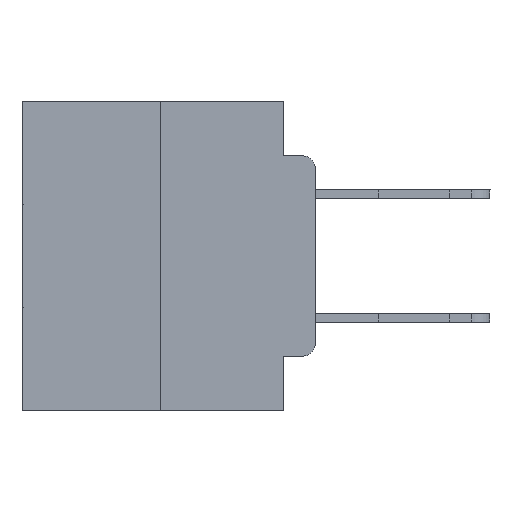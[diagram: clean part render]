
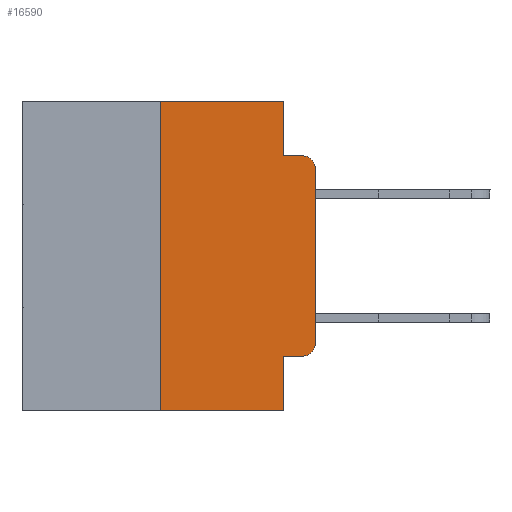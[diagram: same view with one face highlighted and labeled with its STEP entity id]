
A CAD part, left-side view. The second image highlights one B-rep face of the part: STEP entity #16590.
In plain terms, the highlighted planar face has unit normal (-1, 0, 0).
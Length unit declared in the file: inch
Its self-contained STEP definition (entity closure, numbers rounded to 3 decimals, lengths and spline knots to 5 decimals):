
#237 = DIRECTION ( 'NONE',  ( 0., 0., 1. ) ) ;
#585 = CARTESIAN_POINT ( 'NONE',  ( 0., 0.473, 0. ) ) ;
#592 = ORIENTED_EDGE ( 'NONE', *, *, #7788, .T. ) ;
#668 = VERTEX_POINT ( 'NONE', #2514 ) ;
#1977 = VERTEX_POINT ( 'NONE', #4377 ) ;
#2514 = CARTESIAN_POINT ( 'NONE',  ( 0., 0.051, 0. ) ) ;
#2603 = DIRECTION ( 'NONE',  ( 0., -1., 0. ) ) ;
#3077 = ORIENTED_EDGE ( 'NONE', *, *, #17697, .F. ) ;
#4150 = VECTOR ( 'NONE', #15888, 39.37008 ) ;
#4196 = ORIENTED_EDGE ( 'NONE', *, *, #24489, .F. ) ;
#4325 = CARTESIAN_POINT ( 'NONE',  ( 0., 0.051, -0.4115 ) ) ;
#4377 = CARTESIAN_POINT ( 'NONE',  ( 0., 0.25, -0.5 ) ) ;
#4650 = CARTESIAN_POINT ( 'NONE',  ( 0., 0., -0.1085 ) ) ;
#4877 = VERTEX_POINT ( 'NONE', #4325 ) ;
#4922 = LINE ( 'NONE', #20144, #4150 ) ;
#5727 = VERTEX_POINT ( 'NONE', #19335 ) ;
#6522 = DIRECTION ( 'NONE',  ( 0., 0., 1. ) ) ;
#6917 = LINE ( 'NONE', #19869, #20820 ) ;
#7224 = CARTESIAN_POINT ( 'NONE',  ( 0., 0.051, 0. ) ) ;
#7379 = DIRECTION ( 'NONE',  ( 0., 0., -1. ) ) ;
#7439 = CARTESIAN_POINT ( 'NONE',  ( 0., 0.02, -0.4115 ) ) ;
#7537 = EDGE_CURVE ( 'NONE', #4877, #9362, #4922, .T. ) ;
#7606 = CARTESIAN_POINT ( 'NONE',  ( 0., 0.473, -0.5 ) ) ;
#7788 = EDGE_CURVE ( 'NONE', #1977, #18421, #7886, .T. ) ;
#7886 = LINE ( 'NONE', #7606, #14644 ) ;
#8038 = DIRECTION ( 'NONE',  ( 1., 0., 0. ) ) ;
#8735 = EDGE_LOOP ( 'NONE', ( #16158, #27619, #15827, #17125, #17942, #3077, #592, #4196, #11547, #19178 ) ) ;
#9145 = CARTESIAN_POINT ( 'NONE',  ( 0., 0.051, -0.0885 ) ) ;
#9362 = VERTEX_POINT ( 'NONE', #7439 ) ;
#10074 = AXIS2_PLACEMENT_3D ( 'NONE', #19563, #8038, #23288 ) ;
#10873 = FACE_OUTER_BOUND ( 'NONE', #8735, .T. ) ;
#11146 = AXIS2_PLACEMENT_3D ( 'NONE', #19406, #27556, #17004 ) ;
#11332 = EDGE_CURVE ( 'NONE', #9362, #27834, #20157, .T. ) ;
#11547 = ORIENTED_EDGE ( 'NONE', *, *, #7537, .T. ) ;
#11781 = LINE ( 'NONE', #7224, #18985 ) ;
#12015 = VECTOR ( 'NONE', #14668, 39.37008 ) ;
#12826 = LINE ( 'NONE', #19213, #12015 ) ;
#12827 = CARTESIAN_POINT ( 'NONE',  ( 0., 0.02, -0.3915 ) ) ;
#12895 = PLANE ( 'NONE',  #10074 ) ;
#13830 = LINE ( 'NONE', #585, #20642 ) ;
#14644 = VECTOR ( 'NONE', #24995, 39.37008 ) ;
#14668 = DIRECTION ( 'NONE',  ( 0., 0., -1. ) ) ;
#15209 = VERTEX_POINT ( 'NONE', #23945 ) ;
#15827 = ORIENTED_EDGE ( 'NONE', *, *, #17400, .F. ) ;
#15888 = DIRECTION ( 'NONE',  ( 0., -1., 0. ) ) ;
#16083 = AXIS2_PLACEMENT_3D ( 'NONE', #12827, #21492, #28055 ) ;
#16158 = ORIENTED_EDGE ( 'NONE', *, *, #24740, .T. ) ;
#16590 = ADVANCED_FACE ( 'NONE', ( #10873 ), #12895, .F. ) ;
#16642 = VERTEX_POINT ( 'NONE', #24550 ) ;
#17004 = DIRECTION ( 'NONE',  ( 0., 0., -1. ) ) ;
#17076 = CARTESIAN_POINT ( 'NONE',  ( 0., 0.25, 0. ) ) ;
#17125 = ORIENTED_EDGE ( 'NONE', *, *, #19511, .F. ) ;
#17400 = EDGE_CURVE ( 'NONE', #16642, #5727, #26253, .T. ) ;
#17697 = EDGE_CURVE ( 'NONE', #1977, #15209, #19478, .T. ) ;
#17942 = ORIENTED_EDGE ( 'NONE', *, *, #20484, .F. ) ;
#18421 = VERTEX_POINT ( 'NONE', #26441 ) ;
#18985 = VECTOR ( 'NONE', #7379, 39.37008 ) ;
#19178 = ORIENTED_EDGE ( 'NONE', *, *, #11332, .T. ) ;
#19213 = CARTESIAN_POINT ( 'NONE',  ( 0., 0.051, 0. ) ) ;
#19335 = CARTESIAN_POINT ( 'NONE',  ( 0., 0.02, -0.0885 ) ) ;
#19406 = CARTESIAN_POINT ( 'NONE',  ( 0., 0.02, -0.1085 ) ) ;
#19478 = LINE ( 'NONE', #17076, #25613 ) ;
#19511 = EDGE_CURVE ( 'NONE', #668, #16642, #12826, .T. ) ;
#19563 = CARTESIAN_POINT ( 'NONE',  ( 0., 0.473, 0. ) ) ;
#19869 = CARTESIAN_POINT ( 'NONE',  ( 0., 0., 0. ) ) ;
#20089 = DIRECTION ( 'NONE',  ( 0., -1., 0. ) ) ;
#20144 = CARTESIAN_POINT ( 'NONE',  ( 0., 0.051, -0.4115 ) ) ;
#20157 = CIRCLE ( 'NONE', #16083, 0.02 ) ;
#20484 = EDGE_CURVE ( 'NONE', #15209, #668, #13830, .T. ) ;
#20642 = VECTOR ( 'NONE', #20089, 39.37008 ) ;
#20820 = VECTOR ( 'NONE', #237, 39.37008 ) ;
#21292 = VERTEX_POINT ( 'NONE', #4650 ) ;
#21492 = DIRECTION ( 'NONE',  ( -1., 0., 0. ) ) ;
#22249 = EDGE_CURVE ( 'NONE', #21292, #5727, #24811, .T. ) ;
#23288 = DIRECTION ( 'NONE',  ( 0., 0., -1. ) ) ;
#23945 = CARTESIAN_POINT ( 'NONE',  ( 0., 0.25, 0. ) ) ;
#24489 = EDGE_CURVE ( 'NONE', #4877, #18421, #11781, .T. ) ;
#24550 = CARTESIAN_POINT ( 'NONE',  ( 0., 0.051, -0.0885 ) ) ;
#24691 = VECTOR ( 'NONE', #2603, 39.37008 ) ;
#24740 = EDGE_CURVE ( 'NONE', #27834, #21292, #6917, .T. ) ;
#24811 = CIRCLE ( 'NONE', #11146, 0.02 ) ;
#24995 = DIRECTION ( 'NONE',  ( 0., -1., 0. ) ) ;
#25613 = VECTOR ( 'NONE', #6522, 39.37008 ) ;
#26253 = LINE ( 'NONE', #9145, #24691 ) ;
#26441 = CARTESIAN_POINT ( 'NONE',  ( 0., 0.051, -0.5 ) ) ;
#27556 = DIRECTION ( 'NONE',  ( -1., 0., 0. ) ) ;
#27589 = CARTESIAN_POINT ( 'NONE',  ( 0., 0., -0.3915 ) ) ;
#27619 = ORIENTED_EDGE ( 'NONE', *, *, #22249, .T. ) ;
#27834 = VERTEX_POINT ( 'NONE', #27589 ) ;
#28055 = DIRECTION ( 'NONE',  ( 0., 0., -1. ) ) ;
